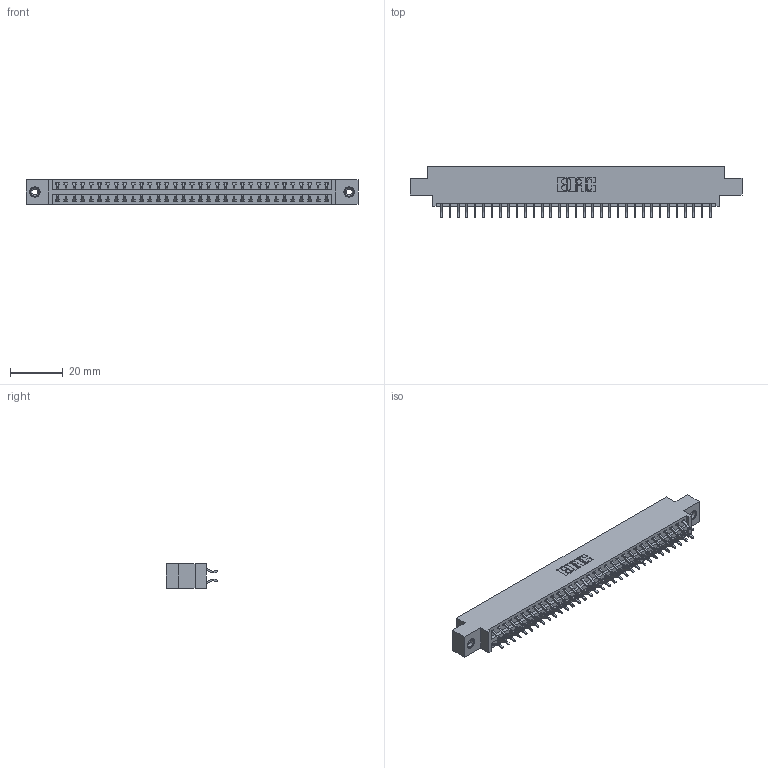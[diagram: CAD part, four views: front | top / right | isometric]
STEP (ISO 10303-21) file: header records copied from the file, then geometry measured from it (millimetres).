
FILE_DESCRIPTION (( 'STEP AP203' ), '1' );
FILE_NAME ('396-066-556-808.STEP', '2018-09-08T19:55:50', ( '' ), ( '' ), 'SwSTEP 2.0', 'SolidWorks 2016', '' );
FILE_SCHEMA (( 'CONFIG_CONTROL_DESIGN' ));
Length unit declared in the file: inch
Products named in the file (4): 346 Part_0.170 Offset - 0.156 Dia-TI; 345-292-001_556 Tail; 345-250-001_345-250-003-102; 396-066-556-808
Assembly tree (69 placements, depth 2):
  396-066-556-808
    346 Part_0.170 Offset - 0.156 Dia-TI
    345-292-001_556 Tail  x66
    345-250-001_345-250-003-102  x2
Bounding box: 125.35 x 19.57 x 9.4 mm (x, y, z)
Volume: 11989.4 mm3; surface area: 16477.2 mm2
Topology: 69 solids, 69 shells, 4014 faces, 11895 edges, 7834 vertices
Faces by surface type: plane 2686, cylinder 1312, cone 12, torus 4
Entity records: 24286 total; most frequent: CARTESIAN_POINT 4015, ORIENTED_EDGE 3930, DIRECTION 3603, EDGE_CURVE 1965, LINE 1673, VECTOR 1673, VERTEX_POINT 1304, AXIS2_PLACEMENT_3D 965
